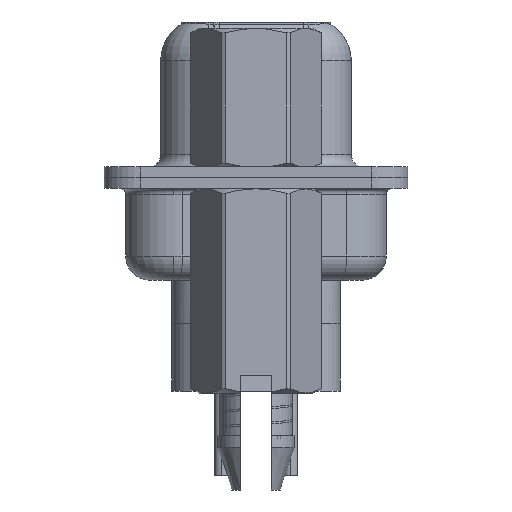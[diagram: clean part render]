
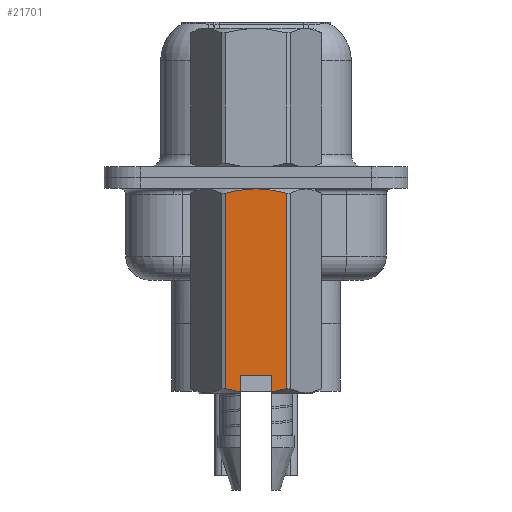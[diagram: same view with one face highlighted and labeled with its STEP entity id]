
A CAD part, left-side view. The second image highlights one B-rep face of the part: STEP entity #21701.
In plain terms, the highlighted planar face has unit normal (-1, 0, 0).
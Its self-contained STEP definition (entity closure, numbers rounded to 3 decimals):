
#2647 = VERTEX_POINT ( 'NONE', #26802 ) ;
#3012 = DIRECTION ( 'NONE',  ( 0., 0., 1. ) ) ;
#3626 = ORIENTED_EDGE ( 'NONE', *, *, #14456, .T. ) ;
#4075 = EDGE_CURVE ( 'NONE', #2647, #17476, #35539, .T. ) ;
#4530 = CARTESIAN_POINT ( 'NONE',  ( -2.381, 1.273, -8.748 ) ) ;
#6733 = CARTESIAN_POINT ( 'NONE',  ( -2.381, -0.428, -0.485 ) ) ;
#6791 = CARTESIAN_POINT ( 'NONE',  ( -2.381, -0.625, -8.885 ) ) ;
#7206 = VECTOR ( 'NONE', #9803, 1000. ) ;
#7329 = EDGE_CURVE ( 'NONE', #8195, #17769, #29469, .T. ) ;
#7715 = DIRECTION ( 'NONE',  ( 0., 0., -1. ) ) ;
#8195 = VERTEX_POINT ( 'NONE', #23491 ) ;
#8520 = EDGE_CURVE ( 'NONE', #14076, #45038, #38567, .T. ) ;
#8969 = VECTOR ( 'NONE', #33670, 1000. ) ;
#9803 = DIRECTION ( 'NONE',  ( 0., 1., 0. ) ) ;
#11246 = LINE ( 'NONE', #25890, #14210 ) ;
#11371 = CARTESIAN_POINT ( 'NONE',  ( -2.381, 0.625, -8.885 ) ) ;
#13346 = CARTESIAN_POINT ( 'NONE',  ( -2.381, -0.853, -0.549 ) ) ;
#14039 = CARTESIAN_POINT ( 'NONE',  ( -2.381, -0.625, -8.2 ) ) ;
#14076 = VERTEX_POINT ( 'NONE', #27811 ) ;
#14210 = VECTOR ( 'NONE', #7715, 1000. ) ;
#14456 = EDGE_CURVE ( 'NONE', #14526, #8195, #40787, .T. ) ;
#14526 = VERTEX_POINT ( 'NONE', #6791 ) ;
#14794 = VECTOR ( 'NONE', #26675, 1000. ) ;
#15360 = EDGE_CURVE ( 'NONE', #16670, #36137, #26084, .T. ) ;
#16670 = VERTEX_POINT ( 'NONE', #19119 ) ;
#16702 = FACE_OUTER_BOUND ( 'NONE', #20863, .T. ) ;
#16933 = CARTESIAN_POINT ( 'NONE',  ( -2.381, 0.625, -8.2 ) ) ;
#17194 = CARTESIAN_POINT ( 'NONE',  ( -2.381, 1.066, -0.596 ) ) ;
#17427 = CARTESIAN_POINT ( 'NONE',  ( -2.381, 0., -0.468 ) ) ;
#17476 = VERTEX_POINT ( 'NONE', #38944 ) ;
#17648 = CARTESIAN_POINT ( 'NONE',  ( -2.381, -1.273, -8.748 ) ) ;
#17656 = EDGE_CURVE ( 'NONE', #36137, #2647, #40594, .T. ) ;
#17769 = VERTEX_POINT ( 'NONE', #22908 ) ;
#18323 = EDGE_CURVE ( 'NONE', #45038, #17476, #43853, .T. ) ;
#18749 = ORIENTED_EDGE ( 'NONE', *, *, #7329, .T. ) ;
#19119 = CARTESIAN_POINT ( 'NONE',  ( -2.381, 0., -0.468 ) ) ;
#19125 = CARTESIAN_POINT ( 'NONE',  ( -2.381, 1.273, 0.581 ) ) ;
#19155 = CARTESIAN_POINT ( 'NONE',  ( -2.381, 0.845, -8.853 ) ) ;
#19636 = VECTOR ( 'NONE', #29706, 1000. ) ;
#20479 = PLANE ( 'NONE',  #42300 ) ;
#20863 = EDGE_LOOP ( 'NONE', ( #32447, #39001, #30883, #3626, #18749, #37922, #44417, #39526, #46063 ) ) ;
#21701 = ADVANCED_FACE ( 'NONE', ( #16702 ), #20479, .T. ) ;
#21893 = CARTESIAN_POINT ( 'NONE',  ( -2.381, -0.625, -8.885 ) ) ;
#22908 = CARTESIAN_POINT ( 'NONE',  ( -2.381, -1.273, -0.652 ) ) ;
#23491 = CARTESIAN_POINT ( 'NONE',  ( -2.381, -1.273, -8.748 ) ) ;
#23975 = CARTESIAN_POINT ( 'NONE',  ( -2.381, 0., -0.468 ) ) ;
#24497 = DIRECTION ( 'NONE',  ( -1., 0., 0. ) ) ;
#24686 = CARTESIAN_POINT ( 'NONE',  ( -2.381, -1.065, -0.596 ) ) ;
#25890 = CARTESIAN_POINT ( 'NONE',  ( -2.381, -0.625, -8.2 ) ) ;
#25945 = CARTESIAN_POINT ( 'NONE',  ( -2.381, -1.273, 0.581 ) ) ;
#26084 = B_SPLINE_CURVE_WITH_KNOTS ( 'NONE', 3,
 ( #17427, #38652, #42902, #27582, #17194, #46463 ),
 .UNSPECIFIED., .F., .F.,
 ( 4, 2, 4 ),
 ( 0.004, 0.004, 0.005 ),
 .UNSPECIFIED. ) ;
#26675 = DIRECTION ( 'NONE',  ( 0., 0., -1. ) ) ;
#26802 = CARTESIAN_POINT ( 'NONE',  ( -2.381, 1.273, -8.748 ) ) ;
#27582 = CARTESIAN_POINT ( 'NONE',  ( -2.381, 0.858, -0.55 ) ) ;
#27811 = CARTESIAN_POINT ( 'NONE',  ( -2.381, -0.625, -8.2 ) ) ;
#28511 = CARTESIAN_POINT ( 'NONE',  ( -2.381, -0.842, -8.854 ) ) ;
#28837 = CARTESIAN_POINT ( 'NONE',  ( -2.381, 1.273, -0.652 ) ) ;
#29469 = LINE ( 'NONE', #25945, #19636 ) ;
#29706 = DIRECTION ( 'NONE',  ( 0., 0., 1. ) ) ;
#30883 = ORIENTED_EDGE ( 'NONE', *, *, #40339, .T. ) ;
#31014 = EDGE_CURVE ( 'NONE', #17769, #16670, #35866, .T. ) ;
#32209 = CARTESIAN_POINT ( 'NONE',  ( -2.381, -0.215, -0.468 ) ) ;
#32447 = ORIENTED_EDGE ( 'NONE', *, *, #18323, .F. ) ;
#32986 = CARTESIAN_POINT ( 'NONE',  ( -2.381, 0.625, -8.2 ) ) ;
#33670 = DIRECTION ( 'NONE',  ( 0., 0., -1. ) ) ;
#35539 = B_SPLINE_CURVE_WITH_KNOTS ( 'NONE', 3,
 ( #4530, #44162, #19155, #11371 ),
 .UNSPECIFIED., .F., .F.,
 ( 4, 4 ),
 ( 0.001, 0.002 ),
 .UNSPECIFIED. ) ;
#35866 = B_SPLINE_CURVE_WITH_KNOTS ( 'NONE', 3,
 ( #42592, #24686, #13346, #6733, #32209, #23975 ),
 .UNSPECIFIED., .F., .F.,
 ( 4, 2, 4 ),
 ( 0.003, 0.003, 0.004 ),
 .UNSPECIFIED. ) ;
#36137 = VERTEX_POINT ( 'NONE', #28837 ) ;
#36259 = CARTESIAN_POINT ( 'NONE',  ( -2.381, -1.06, -8.806 ) ) ;
#37922 = ORIENTED_EDGE ( 'NONE', *, *, #31014, .T. ) ;
#38567 = LINE ( 'NONE', #14039, #7206 ) ;
#38652 = CARTESIAN_POINT ( 'NONE',  ( -2.381, 0.215, -0.468 ) ) ;
#38944 = CARTESIAN_POINT ( 'NONE',  ( -2.381, 0.625, -8.885 ) ) ;
#39001 = ORIENTED_EDGE ( 'NONE', *, *, #8520, .F. ) ;
#39526 = ORIENTED_EDGE ( 'NONE', *, *, #17656, .T. ) ;
#40339 = EDGE_CURVE ( 'NONE', #14076, #14526, #11246, .T. ) ;
#40594 = LINE ( 'NONE', #19125, #14794 ) ;
#40787 = B_SPLINE_CURVE_WITH_KNOTS ( 'NONE', 3,
 ( #21893, #28511, #36259, #17648 ),
 .UNSPECIFIED., .F., .F.,
 ( 4, 4 ),
 ( 0.003, 0.004 ),
 .UNSPECIFIED. ) ;
#42300 = AXIS2_PLACEMENT_3D ( 'NONE', #45969, #24497, #3012 ) ;
#42592 = CARTESIAN_POINT ( 'NONE',  ( -2.381, -1.273, -0.652 ) ) ;
#42902 = CARTESIAN_POINT ( 'NONE',  ( -2.381, 0.432, -0.485 ) ) ;
#43853 = LINE ( 'NONE', #32986, #8969 ) ;
#44162 = CARTESIAN_POINT ( 'NONE',  ( -2.381, 1.06, -8.806 ) ) ;
#44417 = ORIENTED_EDGE ( 'NONE', *, *, #15360, .T. ) ;
#45038 = VERTEX_POINT ( 'NONE', #16933 ) ;
#45969 = CARTESIAN_POINT ( 'NONE',  ( -2.381, -1.375, 7.399 ) ) ;
#46063 = ORIENTED_EDGE ( 'NONE', *, *, #4075, .T. ) ;
#46463 = CARTESIAN_POINT ( 'NONE',  ( -2.381, 1.273, -0.652 ) ) ;
